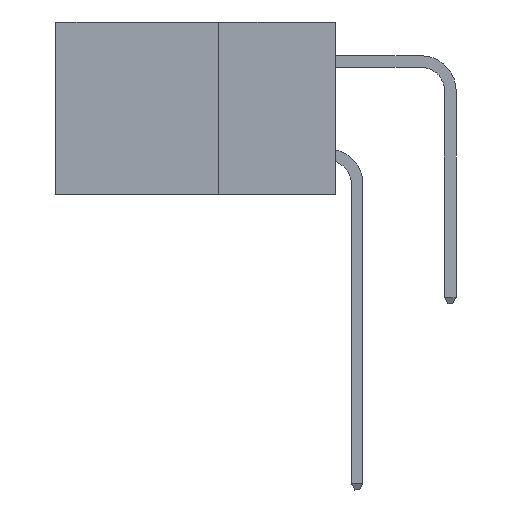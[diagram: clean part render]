
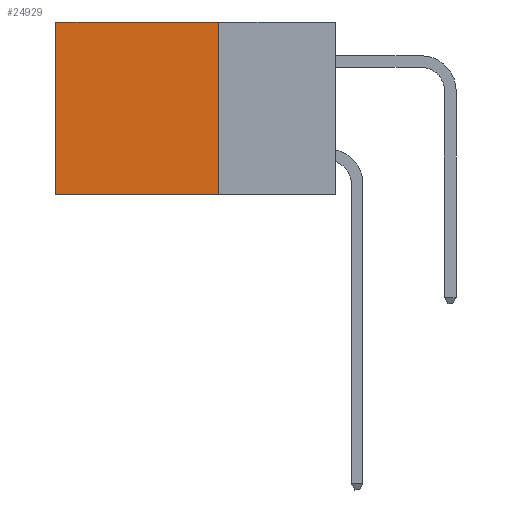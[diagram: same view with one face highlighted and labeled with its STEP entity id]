
A CAD part, left-side view. The second image highlights one B-rep face of the part: STEP entity #24929.
In plain terms, the highlighted planar face has unit normal (-1, 0, 0).
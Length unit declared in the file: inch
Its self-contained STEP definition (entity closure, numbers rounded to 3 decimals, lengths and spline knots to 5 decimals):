
#149 = FACE_OUTER_BOUND ( 'NONE', #13810, .T. ) ;
#1005 = VERTEX_POINT ( 'NONE', #16922 ) ;
#1832 = LINE ( 'NONE', #27094, #17616 ) ;
#1863 = ORIENTED_EDGE ( 'NONE', *, *, #16963, .F. ) ;
#1919 = DIRECTION ( 'NONE',  ( 0., 1., 0. ) ) ;
#1987 = CARTESIAN_POINT ( 'NONE',  ( 0.2875, 0.6, 0. ) ) ;
#4997 = DIRECTION ( 'NONE',  ( 1., 0., 0. ) ) ;
#6327 = EDGE_CURVE ( 'NONE', #1005, #19995, #13485, .T. ) ;
#6906 = CARTESIAN_POINT ( 'NONE',  ( 0.2875, 0.25, 0. ) ) ;
#9736 = DIRECTION ( 'NONE',  ( 0., 1., 0. ) ) ;
#12630 = EDGE_CURVE ( 'NONE', #21529, #19995, #1832, .T. ) ;
#12699 = PLANE ( 'NONE',  #30190 ) ;
#12851 = DIRECTION ( 'NONE',  ( 0., 0., -1. ) ) ;
#13209 = VERTEX_POINT ( 'NONE', #24210 ) ;
#13323 = ORIENTED_EDGE ( 'NONE', *, *, #12630, .F. ) ;
#13485 = LINE ( 'NONE', #1987, #19614 ) ;
#13810 = EDGE_LOOP ( 'NONE', ( #14666, #13323, #1863, #28946 ) ) ;
#14666 = ORIENTED_EDGE ( 'NONE', *, *, #6327, .T. ) ;
#16922 = CARTESIAN_POINT ( 'NONE',  ( 0.2875, 0.6, 0. ) ) ;
#16963 = EDGE_CURVE ( 'NONE', #13209, #21529, #23392, .T. ) ;
#17616 = VECTOR ( 'NONE', #9736, 39.37008 ) ;
#19079 = LINE ( 'NONE', #6906, #31848 ) ;
#19614 = VECTOR ( 'NONE', #12851, 39.37008 ) ;
#19995 = VERTEX_POINT ( 'NONE', #22496 ) ;
#21529 = VERTEX_POINT ( 'NONE', #30811 ) ;
#22496 = CARTESIAN_POINT ( 'NONE',  ( 0.2875, 0.6, -0.37 ) ) ;
#23392 = LINE ( 'NONE', #29391, #32187 ) ;
#24210 = CARTESIAN_POINT ( 'NONE',  ( 0.2875, 0.25, 0. ) ) ;
#24375 = DIRECTION ( 'NONE',  ( 0., 0., -1. ) ) ;
#24929 = ADVANCED_FACE ( 'NONE', ( #149 ), #12699, .F. ) ;
#27094 = CARTESIAN_POINT ( 'NONE',  ( 0.2875, 0.25, -0.37 ) ) ;
#27610 = EDGE_CURVE ( 'NONE', #13209, #1005, #19079, .T. ) ;
#28946 = ORIENTED_EDGE ( 'NONE', *, *, #27610, .T. ) ;
#29391 = CARTESIAN_POINT ( 'NONE',  ( 0.2875, 0.25, 0. ) ) ;
#30190 = AXIS2_PLACEMENT_3D ( 'NONE', #30823, #4997, #33287 ) ;
#30811 = CARTESIAN_POINT ( 'NONE',  ( 0.2875, 0.25, -0.37 ) ) ;
#30823 = CARTESIAN_POINT ( 'NONE',  ( 0.2875, 0.25, 0. ) ) ;
#31848 = VECTOR ( 'NONE', #1919, 39.37008 ) ;
#32187 = VECTOR ( 'NONE', #24375, 39.37008 ) ;
#33287 = DIRECTION ( 'NONE',  ( 0., 0., -1. ) ) ;
